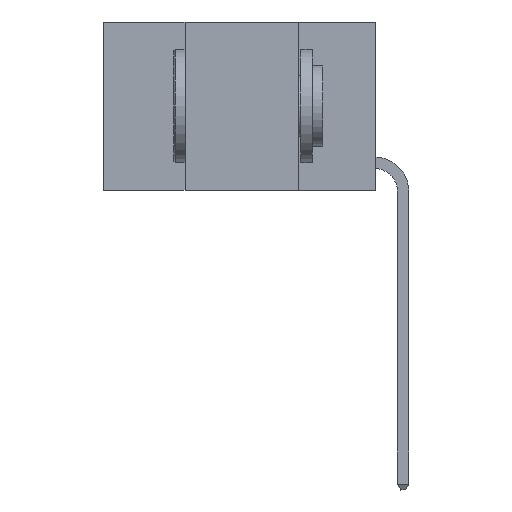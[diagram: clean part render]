
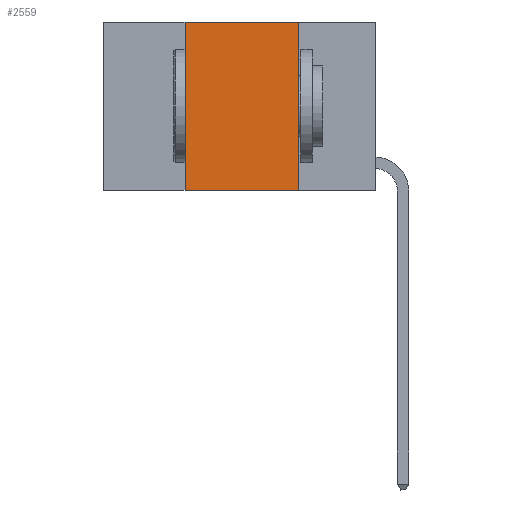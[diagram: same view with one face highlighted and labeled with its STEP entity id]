
A CAD part, left-side view. The second image highlights one B-rep face of the part: STEP entity #2559.
In plain terms, the highlighted planar face has unit normal (-1, 0, 0).
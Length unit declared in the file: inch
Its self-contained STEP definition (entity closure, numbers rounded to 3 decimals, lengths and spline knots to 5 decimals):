
#544 = LINE ( 'NONE', #9381, #17006 ) ;
#1272 = EDGE_LOOP ( 'NONE', ( #17774, #3779, #15127, #17962 ) ) ;
#2559 = ADVANCED_FACE ( 'NONE', ( #7756 ), #3093, .F. ) ;
#3093 = PLANE ( 'NONE',  #10714 ) ;
#3194 = CARTESIAN_POINT ( 'NONE',  ( 0., 0.6, 0. ) ) ;
#3779 = ORIENTED_EDGE ( 'NONE', *, *, #14764, .F. ) ;
#4113 = VECTOR ( 'NONE', #18784, 39.37008 ) ;
#4462 = EDGE_CURVE ( 'NONE', #4907, #12833, #544, .T. ) ;
#4776 = DIRECTION ( 'NONE',  ( 1., 0., 0. ) ) ;
#4907 = VERTEX_POINT ( 'NONE', #7677 ) ;
#5183 = LINE ( 'NONE', #19437, #8745 ) ;
#5691 = CARTESIAN_POINT ( 'NONE',  ( 0., 0.6, 0. ) ) ;
#6403 = EDGE_CURVE ( 'NONE', #18890, #12833, #5183, .T. ) ;
#6709 = CARTESIAN_POINT ( 'NONE',  ( 0., 0.42, 0. ) ) ;
#7677 = CARTESIAN_POINT ( 'NONE',  ( 0., 0.42, -0.37 ) ) ;
#7756 = FACE_OUTER_BOUND ( 'NONE', #1272, .T. ) ;
#8117 = LINE ( 'NONE', #6709, #4113 ) ;
#8745 = VECTOR ( 'NONE', #13592, 39.37008 ) ;
#9042 = DIRECTION ( 'NONE',  ( 0., 0., -1. ) ) ;
#9381 = CARTESIAN_POINT ( 'NONE',  ( 0., 0.6, -0.37 ) ) ;
#10267 = CARTESIAN_POINT ( 'NONE',  ( 0., 0.17, 0. ) ) ;
#10309 = VERTEX_POINT ( 'NONE', #11663 ) ;
#10714 = AXIS2_PLACEMENT_3D ( 'NONE', #3194, #4776, #9042 ) ;
#11663 = CARTESIAN_POINT ( 'NONE',  ( 0., 0.42, 0. ) ) ;
#12832 = EDGE_CURVE ( 'NONE', #4907, #10309, #8117, .T. ) ;
#12833 = VERTEX_POINT ( 'NONE', #15725 ) ;
#13592 = DIRECTION ( 'NONE',  ( 0., 0., -1. ) ) ;
#14764 = EDGE_CURVE ( 'NONE', #10309, #18890, #19452, .T. ) ;
#15127 = ORIENTED_EDGE ( 'NONE', *, *, #12832, .F. ) ;
#15520 = DIRECTION ( 'NONE',  ( 0., -1., 0. ) ) ;
#15725 = CARTESIAN_POINT ( 'NONE',  ( 0., 0.17, -0.37 ) ) ;
#16482 = VECTOR ( 'NONE', #17777, 39.37008 ) ;
#17006 = VECTOR ( 'NONE', #15520, 39.37008 ) ;
#17774 = ORIENTED_EDGE ( 'NONE', *, *, #6403, .F. ) ;
#17777 = DIRECTION ( 'NONE',  ( 0., -1., 0. ) ) ;
#17962 = ORIENTED_EDGE ( 'NONE', *, *, #4462, .T. ) ;
#18784 = DIRECTION ( 'NONE',  ( 0., 0., 1. ) ) ;
#18890 = VERTEX_POINT ( 'NONE', #10267 ) ;
#19437 = CARTESIAN_POINT ( 'NONE',  ( 0., 0.17, 0. ) ) ;
#19452 = LINE ( 'NONE', #5691, #16482 ) ;
